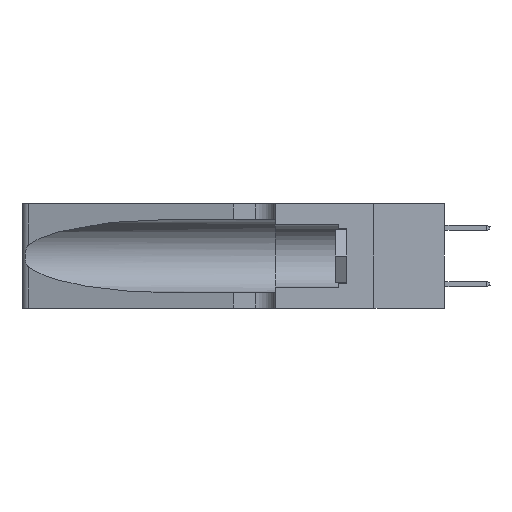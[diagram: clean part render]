
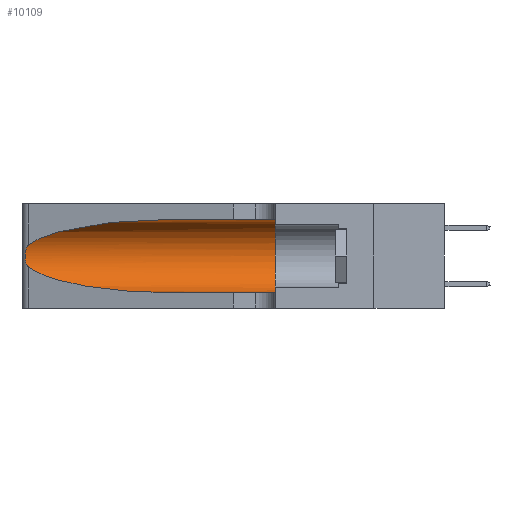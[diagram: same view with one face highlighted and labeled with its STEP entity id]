
A CAD part, left-side view. The second image highlights one B-rep face of the part: STEP entity #10109.
In plain terms, the highlighted cylindrical face has radius 3.308 mm (diameter 6.617 mm), a partial arc.
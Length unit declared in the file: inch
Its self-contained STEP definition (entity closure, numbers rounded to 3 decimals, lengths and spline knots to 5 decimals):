
#168 =( BOUNDED_CURVE ( )  B_SPLINE_CURVE ( 3, ( #6438, #4190, #23130, #8957 ),
 .UNSPECIFIED., .F., .F. ) 
 B_SPLINE_CURVE_WITH_KNOTS ( ( 4, 4 ),
 ( 3.44316, 4.71239 ),
 .UNSPECIFIED. ) 
 CURVE ( )  GEOMETRIC_REPRESENTATION_ITEM ( )  RATIONAL_B_SPLINE_CURVE ( ( 1., 0.87, 0.87, 1. ) ) 
 REPRESENTATION_ITEM ( '' )  );
#867 = VECTOR ( 'NONE', #20166, 39.37008 ) ;
#969 = CARTESIAN_POINT ( 'NONE',  ( 0.1305, 1.61858, 0.31525 ) ) ;
#1327 = CARTESIAN_POINT ( 'NONE',  ( 0.25555, 1.22993, 0.14849 ) ) ;
#1433 = CARTESIAN_POINT ( 'NONE',  ( 0.1305, 0.72297, 0.31525 ) ) ;
#3112 =( BOUNDED_CURVE ( )  B_SPLINE_CURVE ( 3, ( #15993, #27687, #13508, #23082 ),
 .UNSPECIFIED., .F., .T. ) 
 B_SPLINE_CURVE_WITH_KNOTS ( ( 4, 4 ),
 ( 1.5708, 2.84003 ),
 .UNSPECIFIED. ) 
 CURVE ( )  GEOMETRIC_REPRESENTATION_ITEM ( )  RATIONAL_B_SPLINE_CURVE ( ( 1., 0.87, 0.87, 1. ) ) 
 REPRESENTATION_ITEM ( '' )  );
#3562 = CARTESIAN_POINT ( 'NONE',  ( 0.1305, 1.61858, 0.05475 ) ) ;
#3710 = B_SPLINE_CURVE_WITH_KNOTS ( 'NONE', 3,
 ( #29567, #10701, #20256, #6018, #22593, #8423, #24975, #10805, #27298, #13220, #29667, #15605, #1327, #17991 ),
 .UNSPECIFIED., .F., .F.,
 ( 4, 2, 2, 2, 2, 2, 4 ),
 ( 0., 0.00027, 0.00053, 0.00107, 0.0016, 0.00187, 0.00214 ),
 .UNSPECIFIED. ) ;
#4190 = CARTESIAN_POINT ( 'NONE',  ( 0.2373, 1.15595, 0.08982 ) ) ;
#4384 = CARTESIAN_POINT ( 'NONE',  ( 0.1305, 0.35, 0.185 ) ) ;
#4581 = FACE_OUTER_BOUND ( 'NONE', #28971, .T. ) ;
#5222 = EDGE_CURVE ( 'NONE', #26715, #12932, #3112, .T. ) ;
#5741 = CARTESIAN_POINT ( 'NONE',  ( 0.1305, 0.35, 0.31525 ) ) ;
#5749 = VECTOR ( 'NONE', #29420, 39.37008 ) ;
#5875 = CARTESIAN_POINT ( 'NONE',  ( 0.1305, 1.61858, 0.185 ) ) ;
#5976 = DIRECTION ( 'NONE',  ( 0., -1., 0. ) ) ;
#6018 = CARTESIAN_POINT ( 'NONE',  ( 0.25787, 1.23484, 0.2124 ) ) ;
#6438 = CARTESIAN_POINT ( 'NONE',  ( 0.25487, 1.22718, 0.14631 ) ) ;
#6446 = LINE ( 'NONE', #3562, #867 ) ;
#6749 = DIRECTION ( 'NONE',  ( 0., 0., 1. ) ) ;
#8423 = CARTESIAN_POINT ( 'NONE',  ( 0.26018, 1.23835, 0.19895 ) ) ;
#8957 = CARTESIAN_POINT ( 'NONE',  ( 0.1305, 0.72297, 0.05475 ) ) ;
#9079 = ORIENTED_EDGE ( 'NONE', *, *, #26686, .T. ) ;
#10109 = ADVANCED_FACE ( 'NONE', ( #4581 ), #10155, .F. ) ;
#10155 = CYLINDRICAL_SURFACE ( 'NONE', #12779, 0.13025 ) ;
#10231 = VERTEX_POINT ( 'NONE', #11174 ) ;
#10603 = CARTESIAN_POINT ( 'NONE',  ( 0.1305, 0.35, 0.05475 ) ) ;
#10701 = CARTESIAN_POINT ( 'NONE',  ( 0.25555, 1.22994, 0.2215 ) ) ;
#10805 = CARTESIAN_POINT ( 'NONE',  ( 0.26075, 1.23896, 0.178 ) ) ;
#11174 = CARTESIAN_POINT ( 'NONE',  ( 0.1305, 0.72297, 0.05475 ) ) ;
#12779 = AXIS2_PLACEMENT_3D ( 'NONE', #5875, #5976, #29526 ) ;
#12932 = VERTEX_POINT ( 'NONE', #16185 ) ;
#13220 = CARTESIAN_POINT ( 'NONE',  ( 0.25856, 1.23593, 0.16098 ) ) ;
#13508 = CARTESIAN_POINT ( 'NONE',  ( 0.2373, 1.15595, 0.28018 ) ) ;
#15605 = CARTESIAN_POINT ( 'NONE',  ( 0.25639, 1.23186, 0.15144 ) ) ;
#15993 = CARTESIAN_POINT ( 'NONE',  ( 0.1305, 0.72297, 0.31525 ) ) ;
#16185 = CARTESIAN_POINT ( 'NONE',  ( 0.25487, 1.22718, 0.22369 ) ) ;
#16316 = AXIS2_PLACEMENT_3D ( 'NONE', #4384, #20971, #6749 ) ;
#16662 = EDGE_CURVE ( 'NONE', #23995, #10231, #168, .T. ) ;
#17571 = VERTEX_POINT ( 'NONE', #10603 ) ;
#17961 = CIRCLE ( 'NONE', #16316, 0.13025 ) ;
#17991 = CARTESIAN_POINT ( 'NONE',  ( 0.25487, 1.22718, 0.14631 ) ) ;
#18412 = LINE ( 'NONE', #969, #5749 ) ;
#18922 = VERTEX_POINT ( 'NONE', #5741 ) ;
#18965 = ORIENTED_EDGE ( 'NONE', *, *, #25253, .F. ) ;
#19496 = EDGE_CURVE ( 'NONE', #10231, #17571, #6446, .T. ) ;
#20166 = DIRECTION ( 'NONE',  ( 0., -1., 0. ) ) ;
#20256 = CARTESIAN_POINT ( 'NONE',  ( 0.25639, 1.23184, 0.21858 ) ) ;
#20971 = DIRECTION ( 'NONE',  ( 0., 1., 0. ) ) ;
#22593 = CARTESIAN_POINT ( 'NONE',  ( 0.25854, 1.2359, 0.20912 ) ) ;
#23082 = CARTESIAN_POINT ( 'NONE',  ( 0.25487, 1.22718, 0.22369 ) ) ;
#23130 = CARTESIAN_POINT ( 'NONE',  ( 0.18966, 0.96281, 0.05475 ) ) ;
#23181 = CARTESIAN_POINT ( 'NONE',  ( 0.25487, 1.22718, 0.14631 ) ) ;
#23857 = ORIENTED_EDGE ( 'NONE', *, *, #30090, .F. ) ;
#23995 = VERTEX_POINT ( 'NONE', #23181 ) ;
#24975 = CARTESIAN_POINT ( 'NONE',  ( 0.26075, 1.23896, 0.19203 ) ) ;
#25253 = EDGE_CURVE ( 'NONE', #18922, #17571, #17961, .T. ) ;
#25950 = ORIENTED_EDGE ( 'NONE', *, *, #5222, .T. ) ;
#26593 = ORIENTED_EDGE ( 'NONE', *, *, #16662, .T. ) ;
#26686 = EDGE_CURVE ( 'NONE', #12932, #23995, #3710, .T. ) ;
#26715 = VERTEX_POINT ( 'NONE', #1433 ) ;
#27298 = CARTESIAN_POINT ( 'NONE',  ( 0.26017, 1.23833, 0.17102 ) ) ;
#27687 = CARTESIAN_POINT ( 'NONE',  ( 0.18966, 0.96281, 0.31525 ) ) ;
#28971 = EDGE_LOOP ( 'NONE', ( #25950, #9079, #26593, #30180, #18965, #23857 ) ) ;
#29420 = DIRECTION ( 'NONE',  ( 0., -1., 0. ) ) ;
#29526 = DIRECTION ( 'NONE',  ( 0., 0., -1. ) ) ;
#29567 = CARTESIAN_POINT ( 'NONE',  ( 0.25487, 1.22718, 0.22369 ) ) ;
#29667 = CARTESIAN_POINT ( 'NONE',  ( 0.25789, 1.23486, 0.15765 ) ) ;
#30090 = EDGE_CURVE ( 'NONE', #26715, #18922, #18412, .T. ) ;
#30180 = ORIENTED_EDGE ( 'NONE', *, *, #19496, .T. ) ;
